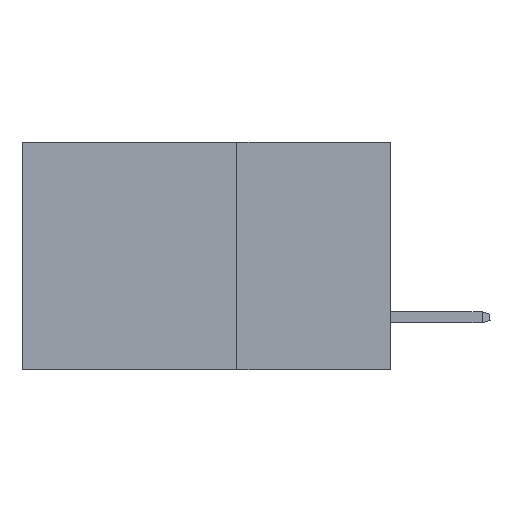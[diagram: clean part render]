
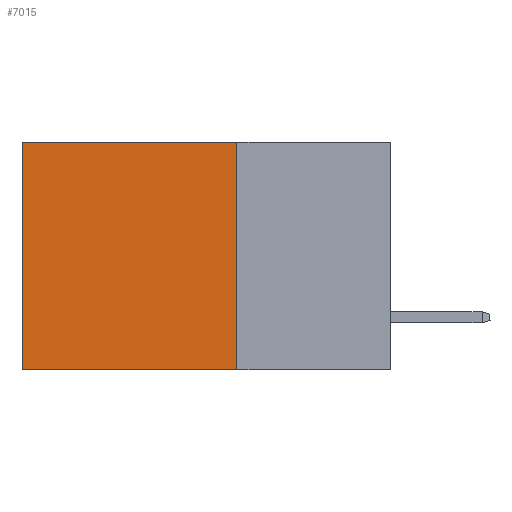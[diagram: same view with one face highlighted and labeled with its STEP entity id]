
A CAD part, left-side view. The second image highlights one B-rep face of the part: STEP entity #7015.
In plain terms, the highlighted planar face has unit normal (-1, 0, 0).
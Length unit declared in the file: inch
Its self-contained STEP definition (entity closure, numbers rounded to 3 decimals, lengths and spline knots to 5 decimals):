
#3458 = CARTESIAN_POINT ( 'NONE',  ( 0.2875, 0.25, 0. ) ) ;
#5536 = DIRECTION ( 'NONE',  ( 0., 0., -1. ) ) ;
#6381 = VECTOR ( 'NONE', #26757, 39.37008 ) ;
#7015 = ADVANCED_FACE ( 'NONE', ( #29532 ), #43655, .F. ) ;
#8854 = CARTESIAN_POINT ( 'NONE',  ( 0.2875, 0.25, 0. ) ) ;
#9898 = CARTESIAN_POINT ( 'NONE',  ( 0.2875, 0.25, -0.37 ) ) ;
#10566 = EDGE_LOOP ( 'NONE', ( #47198, #24101, #47537, #12548 ) ) ;
#10912 = VECTOR ( 'NONE', #25986, 39.37008 ) ;
#11691 = LINE ( 'NONE', #19496, #20855 ) ;
#12548 = ORIENTED_EDGE ( 'NONE', *, *, #16232, .T. ) ;
#14081 = EDGE_CURVE ( 'NONE', #29318, #30282, #11691, .T. ) ;
#16232 = EDGE_CURVE ( 'NONE', #31228, #25979, #21298, .T. ) ;
#16823 = LINE ( 'NONE', #3458, #6381 ) ;
#19496 = CARTESIAN_POINT ( 'NONE',  ( 0.2875, 0.25, -0.37 ) ) ;
#20855 = VECTOR ( 'NONE', #42480, 39.37008 ) ;
#21298 = LINE ( 'NONE', #48818, #10912 ) ;
#23754 = CARTESIAN_POINT ( 'NONE',  ( 0.2875, 0.6, -0.37 ) ) ;
#24101 = ORIENTED_EDGE ( 'NONE', *, *, #14081, .F. ) ;
#24514 = DIRECTION ( 'NONE',  ( 0., 0., -1. ) ) ;
#24944 = CARTESIAN_POINT ( 'NONE',  ( 0.2875, 0.6, 0. ) ) ;
#25979 = VERTEX_POINT ( 'NONE', #44450 ) ;
#25986 = DIRECTION ( 'NONE',  ( 0., 1., 0. ) ) ;
#26757 = DIRECTION ( 'NONE',  ( 0., 0., -1. ) ) ;
#27811 = AXIS2_PLACEMENT_3D ( 'NONE', #8854, #47534, #24514 ) ;
#29318 = VERTEX_POINT ( 'NONE', #9898 ) ;
#29532 = FACE_OUTER_BOUND ( 'NONE', #10566, .T. ) ;
#30282 = VERTEX_POINT ( 'NONE', #23754 ) ;
#31228 = VERTEX_POINT ( 'NONE', #49495 ) ;
#33922 = LINE ( 'NONE', #24944, #42882 ) ;
#42480 = DIRECTION ( 'NONE',  ( 0., 1., 0. ) ) ;
#42882 = VECTOR ( 'NONE', #5536, 39.37008 ) ;
#43332 = EDGE_CURVE ( 'NONE', #31228, #29318, #16823, .T. ) ;
#43655 = PLANE ( 'NONE',  #27811 ) ;
#44450 = CARTESIAN_POINT ( 'NONE',  ( 0.2875, 0.6, 0. ) ) ;
#47198 = ORIENTED_EDGE ( 'NONE', *, *, #49910, .T. ) ;
#47534 = DIRECTION ( 'NONE',  ( 1., 0., 0. ) ) ;
#47537 = ORIENTED_EDGE ( 'NONE', *, *, #43332, .F. ) ;
#48818 = CARTESIAN_POINT ( 'NONE',  ( 0.2875, 0.25, 0. ) ) ;
#49495 = CARTESIAN_POINT ( 'NONE',  ( 0.2875, 0.25, 0. ) ) ;
#49910 = EDGE_CURVE ( 'NONE', #25979, #30282, #33922, .T. ) ;
